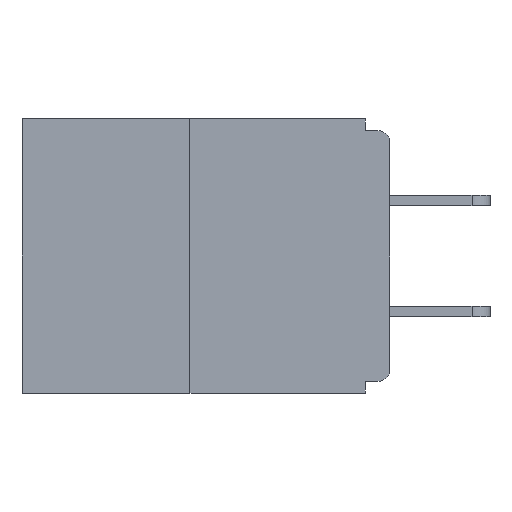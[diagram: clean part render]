
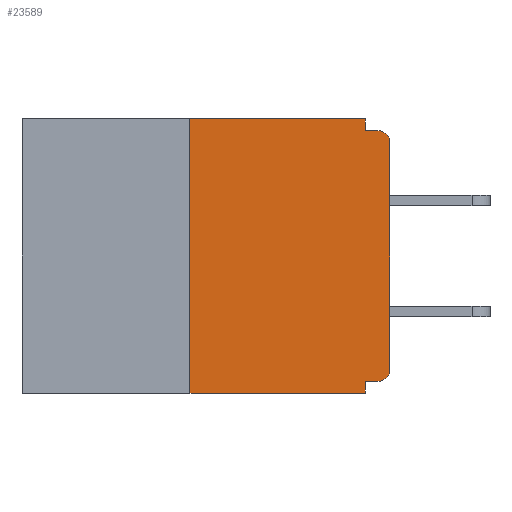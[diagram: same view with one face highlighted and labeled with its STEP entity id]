
A CAD part, left-side view. The second image highlights one B-rep face of the part: STEP entity #23589.
In plain terms, the highlighted planar face has unit normal (-1, 0, 0).
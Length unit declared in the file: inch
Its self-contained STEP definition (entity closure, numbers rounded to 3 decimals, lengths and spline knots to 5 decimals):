
#523 = VECTOR ( 'NONE', #4112, 39.37008 ) ;
#824 = AXIS2_PLACEMENT_3D ( 'NONE', #27094, #24771, #1249 ) ;
#977 = VECTOR ( 'NONE', #20603, 39.37008 ) ;
#1023 = EDGE_CURVE ( 'NONE', #6689, #15720, #20694, .T. ) ;
#1249 = DIRECTION ( 'NONE',  ( 0., 0., -1. ) ) ;
#1358 = ORIENTED_EDGE ( 'NONE', *, *, #1023, .T. ) ;
#1577 = ORIENTED_EDGE ( 'NONE', *, *, #25542, .F. ) ;
#1605 = DIRECTION ( 'NONE',  ( 0., 0., 1. ) ) ;
#1905 = LINE ( 'NONE', #13318, #22920 ) ;
#2324 = CARTESIAN_POINT ( 'NONE',  ( 0., 0.25, 0. ) ) ;
#2592 = DIRECTION ( 'NONE',  ( -1., 0., 0. ) ) ;
#2738 = CARTESIAN_POINT ( 'NONE',  ( 0., 0.031, 0. ) ) ;
#3158 = EDGE_CURVE ( 'NONE', #8803, #18613, #13073, .T. ) ;
#3196 = CARTESIAN_POINT ( 'NONE',  ( 0., 0.031, -0.343 ) ) ;
#3204 = EDGE_CURVE ( 'NONE', #8803, #16047, #1905, .T. ) ;
#3702 = VERTEX_POINT ( 'NONE', #17569 ) ;
#4112 = DIRECTION ( 'NONE',  ( 0., 0., 1. ) ) ;
#4269 = LINE ( 'NONE', #15707, #26007 ) ;
#6015 = PLANE ( 'NONE',  #24358 ) ;
#6198 = ORIENTED_EDGE ( 'NONE', *, *, #3158, .F. ) ;
#6689 = VERTEX_POINT ( 'NONE', #16448 ) ;
#6942 = EDGE_CURVE ( 'NONE', #15720, #20608, #17293, .T. ) ;
#7353 = ORIENTED_EDGE ( 'NONE', *, *, #26026, .F. ) ;
#7447 = EDGE_CURVE ( 'NONE', #20608, #12872, #26364, .T. ) ;
#7511 = DIRECTION ( 'NONE',  ( 0., -1., 0. ) ) ;
#8003 = VERTEX_POINT ( 'NONE', #2738 ) ;
#8330 = CARTESIAN_POINT ( 'NONE',  ( 0., 0.015, -0.015 ) ) ;
#8803 = VERTEX_POINT ( 'NONE', #17522 ) ;
#9558 = VERTEX_POINT ( 'NONE', #16980 ) ;
#9732 = LINE ( 'NONE', #19376, #10765 ) ;
#10389 = ORIENTED_EDGE ( 'NONE', *, *, #11943, .F. ) ;
#10392 = CARTESIAN_POINT ( 'NONE',  ( 0., 0.46, 0. ) ) ;
#10765 = VECTOR ( 'NONE', #27643, 39.37008 ) ;
#11292 = CARTESIAN_POINT ( 'NONE',  ( 0., 0.031, -0.343 ) ) ;
#11405 = ORIENTED_EDGE ( 'NONE', *, *, #6942, .T. ) ;
#11943 = EDGE_CURVE ( 'NONE', #6689, #9558, #24126, .T. ) ;
#11989 = ORIENTED_EDGE ( 'NONE', *, *, #7447, .T. ) ;
#12573 = CARTESIAN_POINT ( 'NONE',  ( 0., 0., 0. ) ) ;
#12836 = LINE ( 'NONE', #3196, #977 ) ;
#12872 = VERTEX_POINT ( 'NONE', #8330 ) ;
#13073 = LINE ( 'NONE', #2324, #523 ) ;
#13318 = CARTESIAN_POINT ( 'NONE',  ( 0., 0.46, -0.343 ) ) ;
#13585 = DIRECTION ( 'NONE',  ( 0., -1., 0. ) ) ;
#15420 = DIRECTION ( 'NONE',  ( 0., -1., 0. ) ) ;
#15707 = CARTESIAN_POINT ( 'NONE',  ( 0., 0., -0.015 ) ) ;
#15720 = VERTEX_POINT ( 'NONE', #21424 ) ;
#16020 = CARTESIAN_POINT ( 'NONE',  ( 0., 0.25, 0. ) ) ;
#16047 = VERTEX_POINT ( 'NONE', #11292 ) ;
#16057 = CARTESIAN_POINT ( 'NONE',  ( 0., 0., -0.03 ) ) ;
#16107 = DIRECTION ( 'NONE',  ( 0., 1., 0. ) ) ;
#16181 = FACE_OUTER_BOUND ( 'NONE', #19550, .T. ) ;
#16448 = CARTESIAN_POINT ( 'NONE',  ( 0., 0.015, -0.328 ) ) ;
#16569 = DIRECTION ( 'NONE',  ( 0., 0., -1. ) ) ;
#16726 = AXIS2_PLACEMENT_3D ( 'NONE', #21871, #2592, #23154 ) ;
#16980 = CARTESIAN_POINT ( 'NONE',  ( 0., 0.031, -0.328 ) ) ;
#17293 = LINE ( 'NONE', #12573, #17629 ) ;
#17522 = CARTESIAN_POINT ( 'NONE',  ( 0., 0.25, -0.343 ) ) ;
#17569 = CARTESIAN_POINT ( 'NONE',  ( 0., 0.031, -0.015 ) ) ;
#17629 = VECTOR ( 'NONE', #1605, 39.37008 ) ;
#17773 = VECTOR ( 'NONE', #7511, 39.37008 ) ;
#17929 = CARTESIAN_POINT ( 'NONE',  ( 0., 0., -0.328 ) ) ;
#18613 = VERTEX_POINT ( 'NONE', #16020 ) ;
#19095 = EDGE_CURVE ( 'NONE', #18613, #8003, #26237, .T. ) ;
#19376 = CARTESIAN_POINT ( 'NONE',  ( 0., 0.031, 0. ) ) ;
#19550 = EDGE_LOOP ( 'NONE', ( #26993, #6198, #22703, #25427, #10389, #1358, #11405, #11989, #7353, #1577 ) ) ;
#20552 = CARTESIAN_POINT ( 'NONE',  ( 0., 0.46, 0. ) ) ;
#20603 = DIRECTION ( 'NONE',  ( 0., 0., -1. ) ) ;
#20608 = VERTEX_POINT ( 'NONE', #16057 ) ;
#20694 = CIRCLE ( 'NONE', #16726, 0.015 ) ;
#21222 = DIRECTION ( 'NONE',  ( 1., 0., 0. ) ) ;
#21424 = CARTESIAN_POINT ( 'NONE',  ( 0., 0., -0.313 ) ) ;
#21871 = CARTESIAN_POINT ( 'NONE',  ( 0., 0.015, -0.313 ) ) ;
#22579 = EDGE_CURVE ( 'NONE', #9558, #16047, #12836, .T. ) ;
#22703 = ORIENTED_EDGE ( 'NONE', *, *, #3204, .T. ) ;
#22770 = VECTOR ( 'NONE', #16107, 39.37008 ) ;
#22920 = VECTOR ( 'NONE', #15420, 39.37008 ) ;
#23154 = DIRECTION ( 'NONE',  ( 0., 0., -1. ) ) ;
#23589 = ADVANCED_FACE ( 'NONE', ( #16181 ), #6015, .F. ) ;
#24126 = LINE ( 'NONE', #17929, #22770 ) ;
#24358 = AXIS2_PLACEMENT_3D ( 'NONE', #10392, #21222, #16569 ) ;
#24771 = DIRECTION ( 'NONE',  ( -1., 0., 0. ) ) ;
#25427 = ORIENTED_EDGE ( 'NONE', *, *, #22579, .F. ) ;
#25542 = EDGE_CURVE ( 'NONE', #8003, #3702, #9732, .T. ) ;
#26007 = VECTOR ( 'NONE', #13585, 39.37008 ) ;
#26026 = EDGE_CURVE ( 'NONE', #3702, #12872, #4269, .T. ) ;
#26237 = LINE ( 'NONE', #20552, #17773 ) ;
#26364 = CIRCLE ( 'NONE', #824, 0.015 ) ;
#26993 = ORIENTED_EDGE ( 'NONE', *, *, #19095, .F. ) ;
#27094 = CARTESIAN_POINT ( 'NONE',  ( 0., 0.015, -0.03 ) ) ;
#27643 = DIRECTION ( 'NONE',  ( 0., 0., -1. ) ) ;
